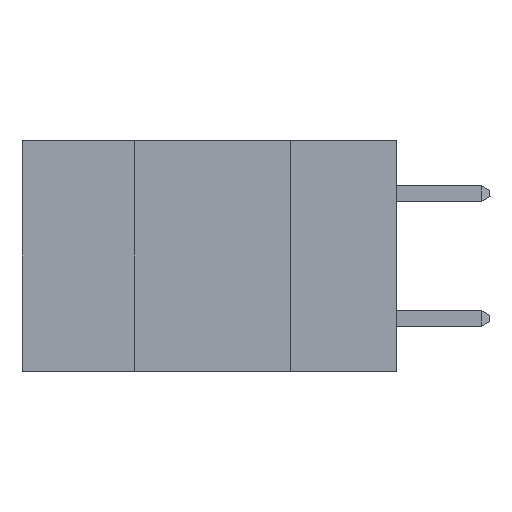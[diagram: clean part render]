
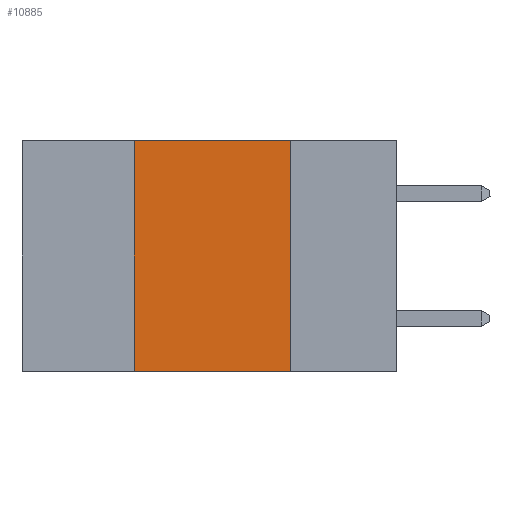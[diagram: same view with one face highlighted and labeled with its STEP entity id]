
A CAD part, left-side view. The second image highlights one B-rep face of the part: STEP entity #10885.
In plain terms, the highlighted planar face has unit normal (-1, 0, 0).
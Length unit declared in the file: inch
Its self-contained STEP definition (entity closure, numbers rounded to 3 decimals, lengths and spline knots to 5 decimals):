
#548 = DIRECTION ( 'NONE',  ( 1., 0., 0. ) ) ;
#980 = DIRECTION ( 'NONE',  ( 0., -1., 0. ) ) ;
#2076 = DIRECTION ( 'NONE',  ( 0., 0., -1. ) ) ;
#2139 = CARTESIAN_POINT ( 'NONE',  ( 0., 0.42, 0. ) ) ;
#2274 = LINE ( 'NONE', #13870, #10501 ) ;
#2430 = CARTESIAN_POINT ( 'NONE',  ( 0., 0.17, 0. ) ) ;
#2803 = VERTEX_POINT ( 'NONE', #2430 ) ;
#3140 = LINE ( 'NONE', #6524, #5526 ) ;
#3592 = EDGE_LOOP ( 'NONE', ( #7686, #4186, #9358, #8154 ) ) ;
#4186 = ORIENTED_EDGE ( 'NONE', *, *, #8603, .F. ) ;
#4603 = VERTEX_POINT ( 'NONE', #10922 ) ;
#5293 = AXIS2_PLACEMENT_3D ( 'NONE', #9223, #548, #13600 ) ;
#5526 = VECTOR ( 'NONE', #11955, 39.37008 ) ;
#6524 = CARTESIAN_POINT ( 'NONE',  ( 0., 0.6, 0. ) ) ;
#7025 = LINE ( 'NONE', #2139, #8522 ) ;
#7686 = ORIENTED_EDGE ( 'NONE', *, *, #9918, .F. ) ;
#8154 = ORIENTED_EDGE ( 'NONE', *, *, #9257, .T. ) ;
#8373 = LINE ( 'NONE', #11692, #11066 ) ;
#8522 = VECTOR ( 'NONE', #11759, 39.37008 ) ;
#8603 = EDGE_CURVE ( 'NONE', #8928, #2803, #3140, .T. ) ;
#8928 = VERTEX_POINT ( 'NONE', #11566 ) ;
#9223 = CARTESIAN_POINT ( 'NONE',  ( 0., 0.6, 0. ) ) ;
#9257 = EDGE_CURVE ( 'NONE', #10722, #4603, #8373, .T. ) ;
#9358 = ORIENTED_EDGE ( 'NONE', *, *, #10012, .F. ) ;
#9901 = CARTESIAN_POINT ( 'NONE',  ( 0., 0.42, -0.37 ) ) ;
#9918 = EDGE_CURVE ( 'NONE', #2803, #4603, #2274, .T. ) ;
#10012 = EDGE_CURVE ( 'NONE', #10722, #8928, #7025, .T. ) ;
#10501 = VECTOR ( 'NONE', #2076, 39.37008 ) ;
#10722 = VERTEX_POINT ( 'NONE', #9901 ) ;
#10885 = ADVANCED_FACE ( 'NONE', ( #13786 ), #11470, .F. ) ;
#10922 = CARTESIAN_POINT ( 'NONE',  ( 0., 0.17, -0.37 ) ) ;
#11066 = VECTOR ( 'NONE', #980, 39.37008 ) ;
#11470 = PLANE ( 'NONE',  #5293 ) ;
#11566 = CARTESIAN_POINT ( 'NONE',  ( 0., 0.42, 0. ) ) ;
#11692 = CARTESIAN_POINT ( 'NONE',  ( 0., 0.6, -0.37 ) ) ;
#11759 = DIRECTION ( 'NONE',  ( 0., 0., 1. ) ) ;
#11955 = DIRECTION ( 'NONE',  ( 0., -1., 0. ) ) ;
#13600 = DIRECTION ( 'NONE',  ( 0., 0., -1. ) ) ;
#13786 = FACE_OUTER_BOUND ( 'NONE', #3592, .T. ) ;
#13870 = CARTESIAN_POINT ( 'NONE',  ( 0., 0.17, 0. ) ) ;
